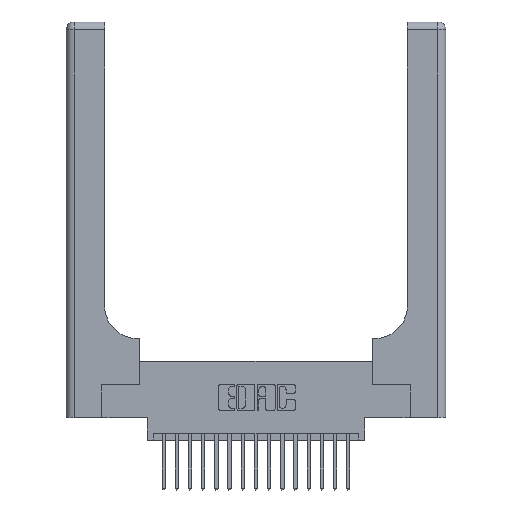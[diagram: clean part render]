
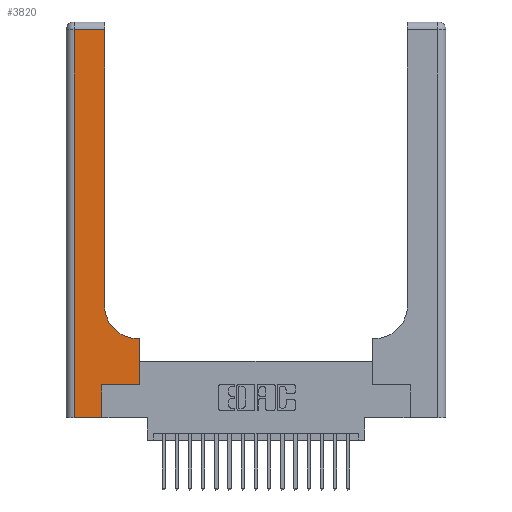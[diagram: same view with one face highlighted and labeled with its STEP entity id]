
A CAD part, top view. The second image highlights one B-rep face of the part: STEP entity #3820.
In plain terms, the highlighted planar face has unit normal (0, 0, 1).
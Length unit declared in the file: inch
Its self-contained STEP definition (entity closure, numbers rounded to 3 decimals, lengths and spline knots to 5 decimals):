
#237 = VECTOR ( 'NONE', #9282, 39.37008 ) ;
#1302 = VERTEX_POINT ( 'NONE', #10411 ) ;
#1314 = VERTEX_POINT ( 'NONE', #10238 ) ;
#1757 = VERTEX_POINT ( 'NONE', #3558 ) ;
#3065 = CARTESIAN_POINT ( 'NONE',  ( 0., 3., 0.37 ) ) ;
#3247 = CARTESIAN_POINT ( 'NONE',  ( 0.06, 3., 0.37 ) ) ;
#3552 = ORIENTED_EDGE ( 'NONE', *, *, #10905, .T. ) ;
#3558 = CARTESIAN_POINT ( 'NONE',  ( 0.5585, 0.6, 0.37 ) ) ;
#3588 = EDGE_CURVE ( 'NONE', #17285, #11812, #18880, .T. ) ;
#3625 = EDGE_CURVE ( 'NONE', #14880, #1314, #9896, .T. ) ;
#3820 = ADVANCED_FACE ( 'NONE', ( #11124 ), #6452, .F. ) ;
#3995 = CARTESIAN_POINT ( 'NONE',  ( 0.5415, 0.85, 0.37 ) ) ;
#4151 = VECTOR ( 'NONE', #6763, 39.37008 ) ;
#4483 = CARTESIAN_POINT ( 'NONE',  ( 0.5585, 0.25, 0.37 ) ) ;
#4605 = LINE ( 'NONE', #3247, #20626 ) ;
#4967 = CIRCLE ( 'NONE', #16827, 0.25 ) ;
#5622 = DIRECTION ( 'NONE',  ( 1., 0., 0. ) ) ;
#5889 = CARTESIAN_POINT ( 'NONE',  ( 0.269, 0., 0.37 ) ) ;
#6335 = EDGE_CURVE ( 'NONE', #1314, #17285, #4605, .T. ) ;
#6339 = LINE ( 'NONE', #6888, #14367 ) ;
#6452 = PLANE ( 'NONE',  #18333 ) ;
#6763 = DIRECTION ( 'NONE',  ( 1., 0., 0. ) ) ;
#6888 = CARTESIAN_POINT ( 'NONE',  ( 0.269, 0., 0.37 ) ) ;
#7115 = ORIENTED_EDGE ( 'NONE', *, *, #19435, .T. ) ;
#7327 = CARTESIAN_POINT ( 'NONE',  ( 0.2915, 0.85, 0.37 ) ) ;
#7448 = VERTEX_POINT ( 'NONE', #14020 ) ;
#7475 = VERTEX_POINT ( 'NONE', #4483 ) ;
#8079 = DIRECTION ( 'NONE',  ( -1., 0., 0. ) ) ;
#8475 = ORIENTED_EDGE ( 'NONE', *, *, #3588, .T. ) ;
#8529 = DIRECTION ( 'NONE',  ( 0., 1., 0. ) ) ;
#8744 = EDGE_CURVE ( 'NONE', #7475, #1757, #12040, .T. ) ;
#8996 = VECTOR ( 'NONE', #16259, 39.37008 ) ;
#9016 = DIRECTION ( 'NONE',  ( -1., 0., 0. ) ) ;
#9282 = DIRECTION ( 'NONE',  ( 0., 1., 0. ) ) ;
#9497 = LINE ( 'NONE', #14636, #8996 ) ;
#9896 = LINE ( 'NONE', #13765, #18385 ) ;
#10143 = EDGE_CURVE ( 'NONE', #7448, #15052, #4967, .T. ) ;
#10238 = CARTESIAN_POINT ( 'NONE',  ( 0.06, 2.94, 0.37 ) ) ;
#10393 = VECTOR ( 'NONE', #18234, 39.37008 ) ;
#10411 = CARTESIAN_POINT ( 'NONE',  ( 0.269, 0.25, 0.37 ) ) ;
#10905 = EDGE_CURVE ( 'NONE', #1302, #7475, #15954, .T. ) ;
#11124 = FACE_OUTER_BOUND ( 'NONE', #19115, .T. ) ;
#11812 = VERTEX_POINT ( 'NONE', #5889 ) ;
#12040 = LINE ( 'NONE', #18831, #237 ) ;
#12190 = ORIENTED_EDGE ( 'NONE', *, *, #10143, .T. ) ;
#12887 = DIRECTION ( 'NONE',  ( 0., -1., 0. ) ) ;
#12980 = CARTESIAN_POINT ( 'NONE',  ( 0.06, 0., 0.37 ) ) ;
#13386 = CARTESIAN_POINT ( 'NONE',  ( 0.2915, 2.94, 0.37 ) ) ;
#13765 = CARTESIAN_POINT ( 'NONE',  ( 0., 2.94, 0.37 ) ) ;
#14020 = CARTESIAN_POINT ( 'NONE',  ( 0.5415, 0.6, 0.37 ) ) ;
#14367 = VECTOR ( 'NONE', #8529, 39.37008 ) ;
#14564 = ORIENTED_EDGE ( 'NONE', *, *, #15425, .T. ) ;
#14636 = CARTESIAN_POINT ( 'NONE',  ( 0.2915, 0.6, 0.37 ) ) ;
#14880 = VERTEX_POINT ( 'NONE', #13386 ) ;
#15052 = VERTEX_POINT ( 'NONE', #7327 ) ;
#15224 = DIRECTION ( 'NONE',  ( 0., 0., -1. ) ) ;
#15425 = EDGE_CURVE ( 'NONE', #11812, #1302, #6339, .T. ) ;
#15954 = LINE ( 'NONE', #16379, #4151 ) ;
#16259 = DIRECTION ( 'NONE',  ( -1., 0., 0. ) ) ;
#16379 = CARTESIAN_POINT ( 'NONE',  ( 0.269, 0.25, 0.37 ) ) ;
#16686 = CARTESIAN_POINT ( 'NONE',  ( 0.2915, 3., 0.37 ) ) ;
#16777 = VECTOR ( 'NONE', #18288, 39.37008 ) ;
#16827 = AXIS2_PLACEMENT_3D ( 'NONE', #3995, #15224, #5622 ) ;
#16830 = ORIENTED_EDGE ( 'NONE', *, *, #3625, .T. ) ;
#17282 = LINE ( 'NONE', #16686, #16777 ) ;
#17285 = VERTEX_POINT ( 'NONE', #12980 ) ;
#17330 = ORIENTED_EDGE ( 'NONE', *, *, #8744, .T. ) ;
#17674 = DIRECTION ( 'NONE',  ( 0., 0., -1. ) ) ;
#18234 = DIRECTION ( 'NONE',  ( 1., 0., 0. ) ) ;
#18288 = DIRECTION ( 'NONE',  ( 0., 1., 0. ) ) ;
#18333 = AXIS2_PLACEMENT_3D ( 'NONE', #3065, #17674, #8079 ) ;
#18385 = VECTOR ( 'NONE', #9016, 39.37008 ) ;
#18773 = EDGE_CURVE ( 'NONE', #15052, #14880, #17282, .T. ) ;
#18831 = CARTESIAN_POINT ( 'NONE',  ( 0.5585, 0.25, 0.37 ) ) ;
#18880 = LINE ( 'NONE', #19775, #10393 ) ;
#19115 = EDGE_LOOP ( 'NONE', ( #19924, #16830, #19766, #8475, #14564, #3552, #17330, #7115, #12190 ) ) ;
#19435 = EDGE_CURVE ( 'NONE', #1757, #7448, #9497, .T. ) ;
#19766 = ORIENTED_EDGE ( 'NONE', *, *, #6335, .T. ) ;
#19775 = CARTESIAN_POINT ( 'NONE',  ( 0., 0., 0.37 ) ) ;
#19924 = ORIENTED_EDGE ( 'NONE', *, *, #18773, .T. ) ;
#20626 = VECTOR ( 'NONE', #12887, 39.37008 ) ;
